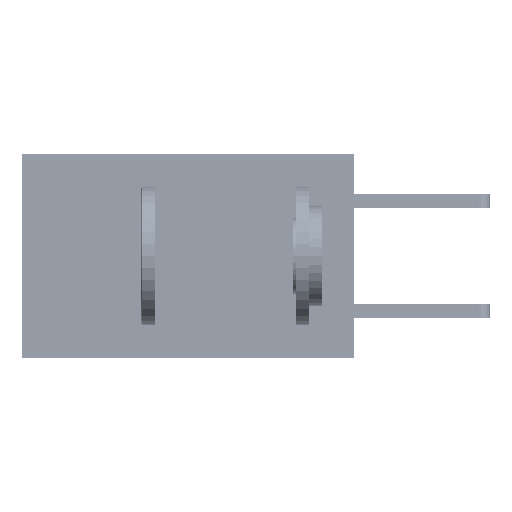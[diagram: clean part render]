
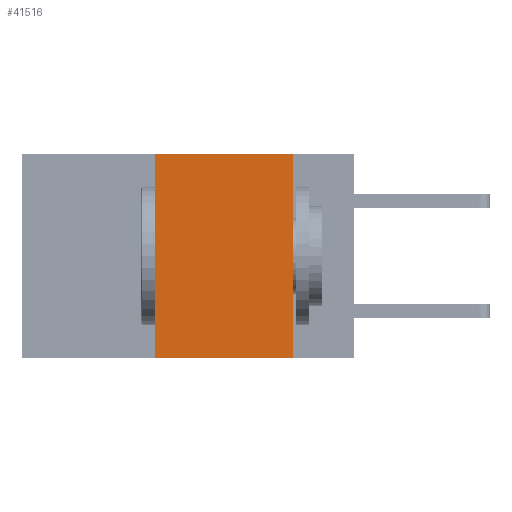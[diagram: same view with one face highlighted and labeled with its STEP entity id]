
A CAD part, left-side view. The second image highlights one B-rep face of the part: STEP entity #41516.
In plain terms, the highlighted planar face has unit normal (-1, 0, 0).
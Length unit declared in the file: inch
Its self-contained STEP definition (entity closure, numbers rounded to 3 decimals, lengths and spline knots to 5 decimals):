
#1559 = PLANE ( 'NONE',  #11306 ) ;
#1729 = CARTESIAN_POINT ( 'NONE',  ( 0., 0.6, 0. ) ) ;
#3596 = CARTESIAN_POINT ( 'NONE',  ( 0., 0.11, -0.37 ) ) ;
#3842 = EDGE_CURVE ( 'NONE', #48194, #7124, #12673, .T. ) ;
#5279 = CARTESIAN_POINT ( 'NONE',  ( 0., 0.36, -0.37 ) ) ;
#7124 = VERTEX_POINT ( 'NONE', #24734 ) ;
#7288 = DIRECTION ( 'NONE',  ( 0., 0., -1. ) ) ;
#7388 = ORIENTED_EDGE ( 'NONE', *, *, #44857, .F. ) ;
#7597 = EDGE_LOOP ( 'NONE', ( #7388, #36977, #31695, #45787 ) ) ;
#9362 = CARTESIAN_POINT ( 'NONE',  ( 0., 0.11, 0. ) ) ;
#9755 = VECTOR ( 'NONE', #15802, 39.37008 ) ;
#11225 = CARTESIAN_POINT ( 'NONE',  ( 0., 0.11, 0. ) ) ;
#11306 = AXIS2_PLACEMENT_3D ( 'NONE', #1729, #16834, #24398 ) ;
#11897 = LINE ( 'NONE', #38789, #42462 ) ;
#12673 = LINE ( 'NONE', #33862, #9755 ) ;
#15802 = DIRECTION ( 'NONE',  ( 0., 0., 1. ) ) ;
#16834 = DIRECTION ( 'NONE',  ( 1., 0., 0. ) ) ;
#17716 = FACE_OUTER_BOUND ( 'NONE', #7597, .T. ) ;
#18199 = LINE ( 'NONE', #11225, #46964 ) ;
#20367 = DIRECTION ( 'NONE',  ( 0., -1., 0. ) ) ;
#22838 = VERTEX_POINT ( 'NONE', #3596 ) ;
#24398 = DIRECTION ( 'NONE',  ( 0., 0., -1. ) ) ;
#24734 = CARTESIAN_POINT ( 'NONE',  ( 0., 0.36, 0. ) ) ;
#26063 = LINE ( 'NONE', #39705, #34873 ) ;
#31695 = ORIENTED_EDGE ( 'NONE', *, *, #3842, .F. ) ;
#32319 = DIRECTION ( 'NONE',  ( 0., -1., 0. ) ) ;
#33862 = CARTESIAN_POINT ( 'NONE',  ( 0., 0.36, 0. ) ) ;
#34873 = VECTOR ( 'NONE', #32319, 39.37008 ) ;
#34970 = EDGE_CURVE ( 'NONE', #7124, #36279, #11897, .T. ) ;
#36279 = VERTEX_POINT ( 'NONE', #9362 ) ;
#36977 = ORIENTED_EDGE ( 'NONE', *, *, #34970, .F. ) ;
#38789 = CARTESIAN_POINT ( 'NONE',  ( 0., 0.6, 0. ) ) ;
#39705 = CARTESIAN_POINT ( 'NONE',  ( 0., 0.6, -0.37 ) ) ;
#41516 = ADVANCED_FACE ( 'NONE', ( #17716 ), #1559, .F. ) ;
#42462 = VECTOR ( 'NONE', #20367, 39.37008 ) ;
#44857 = EDGE_CURVE ( 'NONE', #36279, #22838, #18199, .T. ) ;
#45787 = ORIENTED_EDGE ( 'NONE', *, *, #48268, .T. ) ;
#46964 = VECTOR ( 'NONE', #7288, 39.37008 ) ;
#48194 = VERTEX_POINT ( 'NONE', #5279 ) ;
#48268 = EDGE_CURVE ( 'NONE', #48194, #22838, #26063, .T. ) ;
